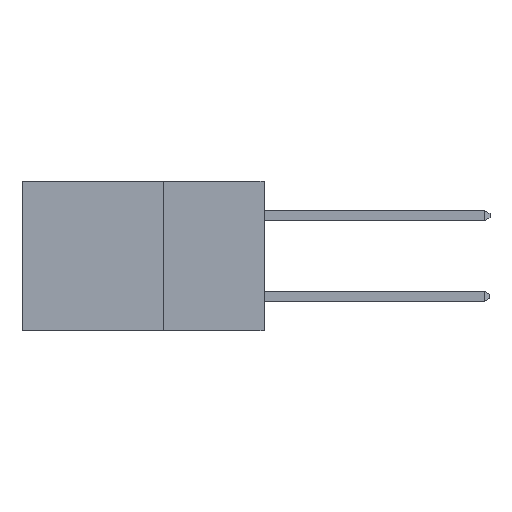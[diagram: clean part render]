
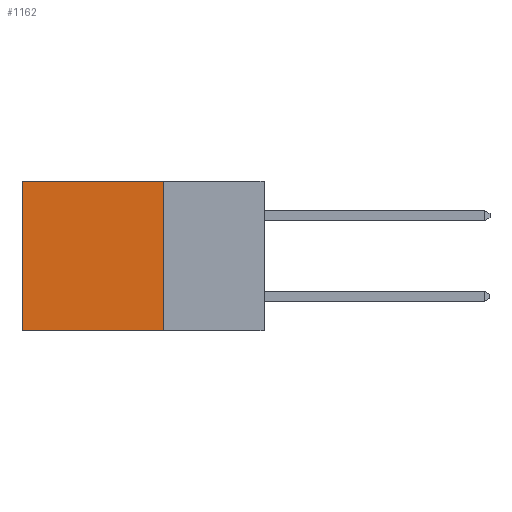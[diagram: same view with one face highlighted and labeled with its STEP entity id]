
A CAD part, left-side view. The second image highlights one B-rep face of the part: STEP entity #1162.
In plain terms, the highlighted planar face has unit normal (-1, 0, 0).
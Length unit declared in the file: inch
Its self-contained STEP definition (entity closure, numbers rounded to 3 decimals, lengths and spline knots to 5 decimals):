
#754 = ORIENTED_EDGE ( 'NONE', *, *, #3863, .F. ) ;
#884 = PLANE ( 'NONE',  #3438 ) ;
#1162 = ADVANCED_FACE ( 'NONE', ( #9316 ), #884, .F. ) ;
#1392 = VECTOR ( 'NONE', #6099, 39.37008 ) ;
#2318 = CARTESIAN_POINT ( 'NONE',  ( 0.2615, 0.6, 0. ) ) ;
#2538 = DIRECTION ( 'NONE',  ( 0., 0., -1. ) ) ;
#2742 = DIRECTION ( 'NONE',  ( 0., 1., 0. ) ) ;
#2803 = LINE ( 'NONE', #7846, #1392 ) ;
#2873 = LINE ( 'NONE', #3797, #4236 ) ;
#3348 = CARTESIAN_POINT ( 'NONE',  ( 0.2615, 0.25, -0.37 ) ) ;
#3438 = AXIS2_PLACEMENT_3D ( 'NONE', #3348, #4175, #2538 ) ;
#3797 = CARTESIAN_POINT ( 'NONE',  ( 0.2615, 0.25, 0. ) ) ;
#3839 = VERTEX_POINT ( 'NONE', #10225 ) ;
#3857 = VECTOR ( 'NONE', #9348, 39.37008 ) ;
#3863 = EDGE_CURVE ( 'NONE', #3839, #7385, #2803, .T. ) ;
#4175 = DIRECTION ( 'NONE',  ( 1., 0., 0. ) ) ;
#4236 = VECTOR ( 'NONE', #6219, 39.37008 ) ;
#4254 = EDGE_CURVE ( 'NONE', #7385, #8666, #7837, .T. ) ;
#4282 = EDGE_CURVE ( 'NONE', #9785, #8666, #7024, .T. ) ;
#5062 = ORIENTED_EDGE ( 'NONE', *, *, #4254, .F. ) ;
#5158 = CARTESIAN_POINT ( 'NONE',  ( 0.2615, 0.6, -0.37 ) ) ;
#5200 = CARTESIAN_POINT ( 'NONE',  ( 0.2615, 0.6, -0.37 ) ) ;
#5667 = ORIENTED_EDGE ( 'NONE', *, *, #8319, .T. ) ;
#5967 = VECTOR ( 'NONE', #2742, 39.37008 ) ;
#6054 = EDGE_LOOP ( 'NONE', ( #7954, #5062, #754, #5667 ) ) ;
#6099 = DIRECTION ( 'NONE',  ( 0., 0., -1. ) ) ;
#6219 = DIRECTION ( 'NONE',  ( 0., 1., 0. ) ) ;
#7024 = LINE ( 'NONE', #5200, #3857 ) ;
#7030 = CARTESIAN_POINT ( 'NONE',  ( 0.2615, 0.25, -0.37 ) ) ;
#7385 = VERTEX_POINT ( 'NONE', #7030 ) ;
#7837 = LINE ( 'NONE', #7888, #5967 ) ;
#7846 = CARTESIAN_POINT ( 'NONE',  ( 0.2615, 0.25, -0.37 ) ) ;
#7888 = CARTESIAN_POINT ( 'NONE',  ( 0.2615, 0.25, -0.37 ) ) ;
#7954 = ORIENTED_EDGE ( 'NONE', *, *, #4282, .T. ) ;
#8319 = EDGE_CURVE ( 'NONE', #3839, #9785, #2873, .T. ) ;
#8666 = VERTEX_POINT ( 'NONE', #5158 ) ;
#9316 = FACE_OUTER_BOUND ( 'NONE', #6054, .T. ) ;
#9348 = DIRECTION ( 'NONE',  ( 0., 0., -1. ) ) ;
#9785 = VERTEX_POINT ( 'NONE', #2318 ) ;
#10225 = CARTESIAN_POINT ( 'NONE',  ( 0.2615, 0.25, 0. ) ) ;
